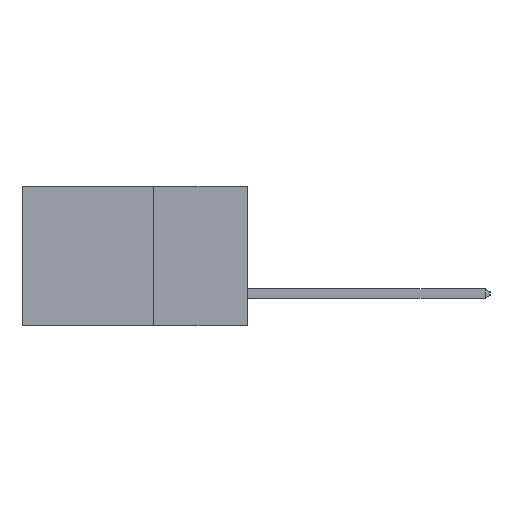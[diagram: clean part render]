
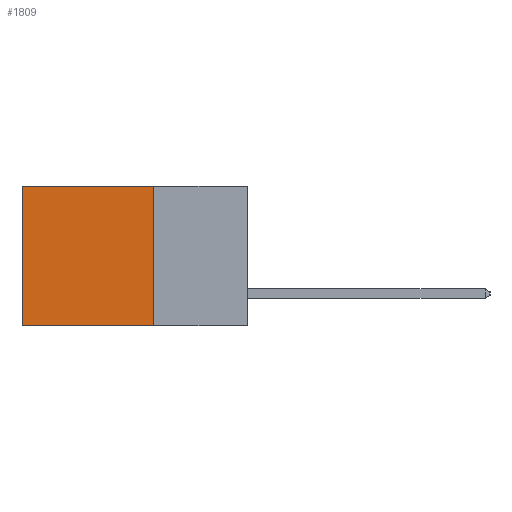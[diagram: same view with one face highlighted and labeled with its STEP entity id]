
A CAD part, left-side view. The second image highlights one B-rep face of the part: STEP entity #1809.
In plain terms, the highlighted planar face has unit normal (-1, 0, 0).
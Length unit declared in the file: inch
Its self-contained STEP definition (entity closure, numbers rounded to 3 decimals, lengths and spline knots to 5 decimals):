
#939 = CARTESIAN_POINT ( 'NONE',  ( 0.2615, 0.25, -0.37 ) ) ;
#1183 = CARTESIAN_POINT ( 'NONE',  ( 0.2615, 0.6, -0.37 ) ) ;
#1679 = LINE ( 'NONE', #10551, #8971 ) ;
#1809 = ADVANCED_FACE ( 'NONE', ( #9637 ), #6771, .F. ) ;
#2120 = EDGE_LOOP ( 'NONE', ( #8016, #7961, #8051, #8079 ) ) ;
#3015 = VERTEX_POINT ( 'NONE', #5030 ) ;
#3374 = EDGE_CURVE ( 'NONE', #3015, #10170, #1679, .T. ) ;
#4091 = VECTOR ( 'NONE', #7719, 39.37008 ) ;
#4621 = CARTESIAN_POINT ( 'NONE',  ( 0.2615, 0.6, -0.37 ) ) ;
#5030 = CARTESIAN_POINT ( 'NONE',  ( 0.2615, 0.25, 0. ) ) ;
#5080 = DIRECTION ( 'NONE',  ( 0., 1., 0. ) ) ;
#5388 = VERTEX_POINT ( 'NONE', #4621 ) ;
#5442 = DIRECTION ( 'NONE',  ( 0., 1., 0. ) ) ;
#6069 = VECTOR ( 'NONE', #11472, 39.37008 ) ;
#6347 = EDGE_CURVE ( 'NONE', #11027, #5388, #10287, .T. ) ;
#6357 = LINE ( 'NONE', #7299, #6069 ) ;
#6472 = DIRECTION ( 'NONE',  ( 0., 0., -1. ) ) ;
#6497 = DIRECTION ( 'NONE',  ( 1., 0., 0. ) ) ;
#6771 = PLANE ( 'NONE',  #9299 ) ;
#6954 = CARTESIAN_POINT ( 'NONE',  ( 0.2615, 0.25, -0.37 ) ) ;
#7073 = EDGE_CURVE ( 'NONE', #10170, #5388, #8484, .T. ) ;
#7299 = CARTESIAN_POINT ( 'NONE',  ( 0.2615, 0.25, -0.37 ) ) ;
#7459 = CARTESIAN_POINT ( 'NONE',  ( 0.2615, 0.6, 0. ) ) ;
#7719 = DIRECTION ( 'NONE',  ( 0., 0., -1. ) ) ;
#7961 = ORIENTED_EDGE ( 'NONE', *, *, #6347, .F. ) ;
#8016 = ORIENTED_EDGE ( 'NONE', *, *, #7073, .T. ) ;
#8051 = ORIENTED_EDGE ( 'NONE', *, *, #10010, .F. ) ;
#8079 = ORIENTED_EDGE ( 'NONE', *, *, #3374, .T. ) ;
#8084 = VECTOR ( 'NONE', #5080, 39.37008 ) ;
#8484 = LINE ( 'NONE', #1183, #4091 ) ;
#8971 = VECTOR ( 'NONE', #5442, 39.37008 ) ;
#9299 = AXIS2_PLACEMENT_3D ( 'NONE', #6954, #6497, #6472 ) ;
#9637 = FACE_OUTER_BOUND ( 'NONE', #2120, .T. ) ;
#10010 = EDGE_CURVE ( 'NONE', #3015, #11027, #6357, .T. ) ;
#10170 = VERTEX_POINT ( 'NONE', #7459 ) ;
#10287 = LINE ( 'NONE', #11025, #8084 ) ;
#10551 = CARTESIAN_POINT ( 'NONE',  ( 0.2615, 0.25, 0. ) ) ;
#11025 = CARTESIAN_POINT ( 'NONE',  ( 0.2615, 0.25, -0.37 ) ) ;
#11027 = VERTEX_POINT ( 'NONE', #939 ) ;
#11472 = DIRECTION ( 'NONE',  ( 0., 0., -1. ) ) ;
